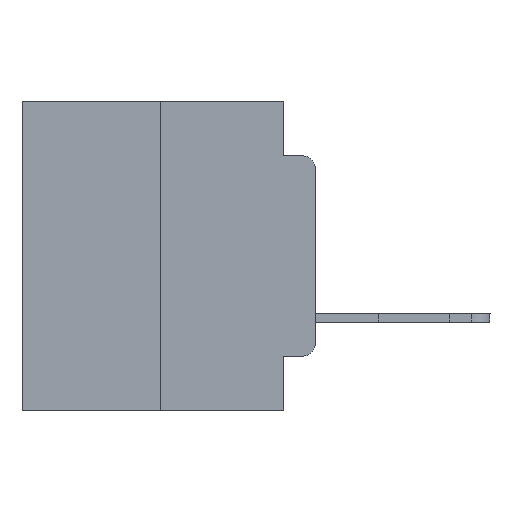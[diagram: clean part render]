
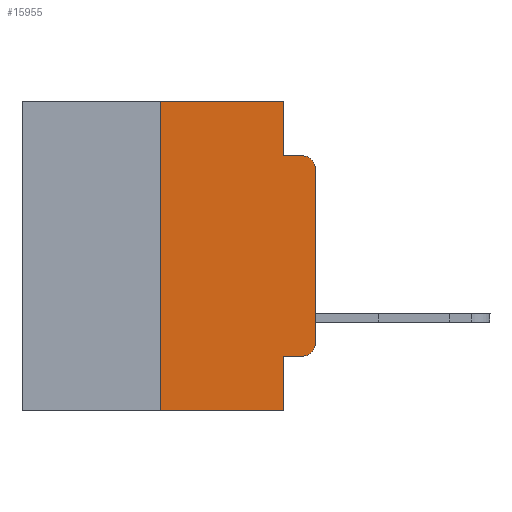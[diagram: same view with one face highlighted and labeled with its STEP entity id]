
A CAD part, left-side view. The second image highlights one B-rep face of the part: STEP entity #15955.
In plain terms, the highlighted planar face has unit normal (-1, 0, 0).
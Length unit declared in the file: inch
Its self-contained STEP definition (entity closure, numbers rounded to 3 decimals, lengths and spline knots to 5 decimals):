
#116 = EDGE_CURVE ( 'NONE', #596, #16930, #9129, .T. ) ;
#596 = VERTEX_POINT ( 'NONE', #3049 ) ;
#955 = DIRECTION ( 'NONE',  ( 0., 0., -1. ) ) ;
#1124 = VERTEX_POINT ( 'NONE', #14414 ) ;
#1706 = CARTESIAN_POINT ( 'NONE',  ( 0., 0.25, -0.5 ) ) ;
#2016 = AXIS2_PLACEMENT_3D ( 'NONE', #12120, #14155, #4304 ) ;
#2452 = CARTESIAN_POINT ( 'NONE',  ( 0., 0.051, -0.4115 ) ) ;
#3023 = VECTOR ( 'NONE', #14614, 39.37008 ) ;
#3049 = CARTESIAN_POINT ( 'NONE',  ( 0., 0.25, 0. ) ) ;
#3341 = DIRECTION ( 'NONE',  ( 0., 0., -1. ) ) ;
#3348 = EDGE_CURVE ( 'NONE', #17657, #1124, #17827, .T. ) ;
#3420 = EDGE_CURVE ( 'NONE', #17657, #23133, #10848, .T. ) ;
#3647 = LINE ( 'NONE', #20035, #13382 ) ;
#4304 = DIRECTION ( 'NONE',  ( 0., 0., -1. ) ) ;
#4635 = DIRECTION ( 'NONE',  ( 0., -1., 0. ) ) ;
#4886 = VECTOR ( 'NONE', #6166, 39.37008 ) ;
#5254 = ORIENTED_EDGE ( 'NONE', *, *, #11550, .T. ) ;
#5277 = CARTESIAN_POINT ( 'NONE',  ( 0., 0.25, 0. ) ) ;
#5471 = VECTOR ( 'NONE', #13179, 39.37008 ) ;
#6140 = AXIS2_PLACEMENT_3D ( 'NONE', #9002, #19184, #955 ) ;
#6166 = DIRECTION ( 'NONE',  ( 0., 0., -1. ) ) ;
#6231 = EDGE_CURVE ( 'NONE', #23133, #8297, #24161, .T. ) ;
#6750 = ORIENTED_EDGE ( 'NONE', *, *, #15665, .F. ) ;
#6886 = EDGE_CURVE ( 'NONE', #19641, #25082, #9243, .T. ) ;
#7507 = ORIENTED_EDGE ( 'NONE', *, *, #116, .F. ) ;
#7948 = VECTOR ( 'NONE', #12197, 39.37008 ) ;
#8006 = EDGE_LOOP ( 'NONE', ( #19685, #5254, #22116, #17717, #7507, #6750, #14679, #11236, #16863, #22301 ) ) ;
#8297 = VERTEX_POINT ( 'NONE', #11129 ) ;
#8411 = CARTESIAN_POINT ( 'NONE',  ( 0., 0., -0.1085 ) ) ;
#9002 = CARTESIAN_POINT ( 'NONE',  ( 0., 0.02, -0.1085 ) ) ;
#9129 = LINE ( 'NONE', #23317, #15473 ) ;
#9243 = LINE ( 'NONE', #10580, #19388 ) ;
#9501 = FACE_OUTER_BOUND ( 'NONE', #8006, .T. ) ;
#9861 = DIRECTION ( 'NONE',  ( 0., 0., 1. ) ) ;
#10050 = CARTESIAN_POINT ( 'NONE',  ( 0., 0.051, -0.0885 ) ) ;
#10458 = CARTESIAN_POINT ( 'NONE',  ( 0., 0.051, -0.4115 ) ) ;
#10580 = CARTESIAN_POINT ( 'NONE',  ( 0., 0.051, -0.0885 ) ) ;
#10798 = LINE ( 'NONE', #5277, #5471 ) ;
#10848 = LINE ( 'NONE', #10458, #3023 ) ;
#11129 = CARTESIAN_POINT ( 'NONE',  ( 0., 0., -0.3915 ) ) ;
#11236 = ORIENTED_EDGE ( 'NONE', *, *, #3348, .F. ) ;
#11550 = EDGE_CURVE ( 'NONE', #24067, #25082, #25864, .T. ) ;
#12120 = CARTESIAN_POINT ( 'NONE',  ( 0., 0.473, 0. ) ) ;
#12197 = DIRECTION ( 'NONE',  ( 0., -1., 0. ) ) ;
#12226 = CARTESIAN_POINT ( 'NONE',  ( 0., 0.051, 0. ) ) ;
#12739 = AXIS2_PLACEMENT_3D ( 'NONE', #15261, #19228, #21281 ) ;
#12892 = EDGE_CURVE ( 'NONE', #16930, #19641, #18870, .T. ) ;
#13179 = DIRECTION ( 'NONE',  ( 0., 0., 1. ) ) ;
#13382 = VECTOR ( 'NONE', #9861, 39.37008 ) ;
#14075 = CARTESIAN_POINT ( 'NONE',  ( 0., 0.473, -0.5 ) ) ;
#14110 = CARTESIAN_POINT ( 'NONE',  ( 0., 0.051, 0. ) ) ;
#14155 = DIRECTION ( 'NONE',  ( 1., 0., 0. ) ) ;
#14414 = CARTESIAN_POINT ( 'NONE',  ( 0., 0.051, -0.5 ) ) ;
#14614 = DIRECTION ( 'NONE',  ( 0., -1., 0. ) ) ;
#14679 = ORIENTED_EDGE ( 'NONE', *, *, #15907, .T. ) ;
#15261 = CARTESIAN_POINT ( 'NONE',  ( 0., 0.02, -0.3915 ) ) ;
#15294 = DIRECTION ( 'NONE',  ( 0., -1., 0. ) ) ;
#15473 = VECTOR ( 'NONE', #15294, 39.37008 ) ;
#15665 = EDGE_CURVE ( 'NONE', #18750, #596, #10798, .T. ) ;
#15907 = EDGE_CURVE ( 'NONE', #18750, #1124, #17128, .T. ) ;
#15955 = ADVANCED_FACE ( 'NONE', ( #9501 ), #24228, .F. ) ;
#16740 = EDGE_CURVE ( 'NONE', #8297, #24067, #3647, .T. ) ;
#16863 = ORIENTED_EDGE ( 'NONE', *, *, #3420, .T. ) ;
#16930 = VERTEX_POINT ( 'NONE', #12226 ) ;
#16970 = VECTOR ( 'NONE', #3341, 39.37008 ) ;
#17128 = LINE ( 'NONE', #14075, #7948 ) ;
#17657 = VERTEX_POINT ( 'NONE', #2452 ) ;
#17717 = ORIENTED_EDGE ( 'NONE', *, *, #12892, .F. ) ;
#17827 = LINE ( 'NONE', #14110, #4886 ) ;
#18750 = VERTEX_POINT ( 'NONE', #1706 ) ;
#18870 = LINE ( 'NONE', #21552, #16970 ) ;
#19184 = DIRECTION ( 'NONE',  ( -1., 0., 0. ) ) ;
#19228 = DIRECTION ( 'NONE',  ( -1., 0., 0. ) ) ;
#19388 = VECTOR ( 'NONE', #4635, 39.37008 ) ;
#19610 = CARTESIAN_POINT ( 'NONE',  ( 0., 0.02, -0.0885 ) ) ;
#19641 = VERTEX_POINT ( 'NONE', #10050 ) ;
#19685 = ORIENTED_EDGE ( 'NONE', *, *, #16740, .T. ) ;
#20035 = CARTESIAN_POINT ( 'NONE',  ( 0., 0., 0. ) ) ;
#21281 = DIRECTION ( 'NONE',  ( 0., 0., -1. ) ) ;
#21552 = CARTESIAN_POINT ( 'NONE',  ( 0., 0.051, 0. ) ) ;
#22116 = ORIENTED_EDGE ( 'NONE', *, *, #6886, .F. ) ;
#22301 = ORIENTED_EDGE ( 'NONE', *, *, #6231, .T. ) ;
#23133 = VERTEX_POINT ( 'NONE', #23189 ) ;
#23189 = CARTESIAN_POINT ( 'NONE',  ( 0., 0.02, -0.4115 ) ) ;
#23317 = CARTESIAN_POINT ( 'NONE',  ( 0., 0.473, 0. ) ) ;
#24067 = VERTEX_POINT ( 'NONE', #8411 ) ;
#24161 = CIRCLE ( 'NONE', #12739, 0.02 ) ;
#24228 = PLANE ( 'NONE',  #2016 ) ;
#25082 = VERTEX_POINT ( 'NONE', #19610 ) ;
#25864 = CIRCLE ( 'NONE', #6140, 0.02 ) ;
